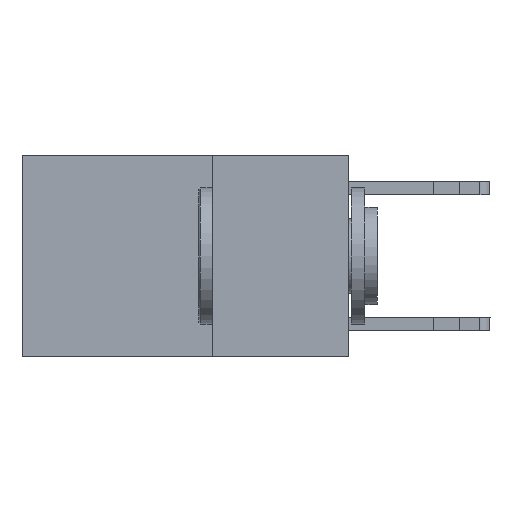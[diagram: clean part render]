
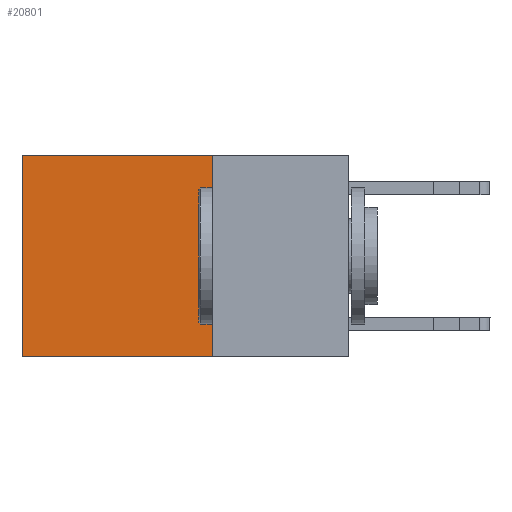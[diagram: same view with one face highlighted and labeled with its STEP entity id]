
A CAD part, left-side view. The second image highlights one B-rep face of the part: STEP entity #20801.
In plain terms, the highlighted planar face has unit normal (-1, 0, 0).
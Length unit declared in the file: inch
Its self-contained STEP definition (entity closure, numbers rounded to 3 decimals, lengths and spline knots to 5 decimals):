
#813 = ORIENTED_EDGE ( 'NONE', *, *, #5533, .F. ) ;
#1489 = VECTOR ( 'NONE', #18342, 39.37008 ) ;
#2137 = LINE ( 'NONE', #18968, #1489 ) ;
#3173 = VECTOR ( 'NONE', #22518, 39.37008 ) ;
#3373 = LINE ( 'NONE', #22597, #3173 ) ;
#4511 = CARTESIAN_POINT ( 'NONE',  ( 0.2625, 0.6, -0.37 ) ) ;
#5533 = EDGE_CURVE ( 'NONE', #21142, #20079, #14805, .T. ) ;
#5697 = CARTESIAN_POINT ( 'NONE',  ( 0.2625, 0.25, 0. ) ) ;
#5754 = DIRECTION ( 'NONE',  ( 0., 1., 0. ) ) ;
#5959 = EDGE_LOOP ( 'NONE', ( #14165, #813, #18058, #15944 ) ) ;
#6231 = CARTESIAN_POINT ( 'NONE',  ( 0.2625, 0.25, -0.37 ) ) ;
#6402 = FACE_OUTER_BOUND ( 'NONE', #5959, .T. ) ;
#8987 = CARTESIAN_POINT ( 'NONE',  ( 0.2625, 0.25, -0.37 ) ) ;
#12621 = VECTOR ( 'NONE', #21147, 39.37008 ) ;
#12795 = LINE ( 'NONE', #20859, #12621 ) ;
#14165 = ORIENTED_EDGE ( 'NONE', *, *, #17484, .T. ) ;
#14754 = VECTOR ( 'NONE', #5754, 39.37008 ) ;
#14805 = LINE ( 'NONE', #6231, #14754 ) ;
#15431 = EDGE_CURVE ( 'NONE', #21270, #23002, #3373, .T. ) ;
#15872 = CARTESIAN_POINT ( 'NONE',  ( 0.2625, 0.6, 0. ) ) ;
#15944 = ORIENTED_EDGE ( 'NONE', *, *, #15431, .T. ) ;
#16678 = EDGE_CURVE ( 'NONE', #21270, #21142, #12795, .T. ) ;
#17484 = EDGE_CURVE ( 'NONE', #23002, #20079, #2137, .T. ) ;
#17991 = DIRECTION ( 'NONE',  ( 0., 0., -1. ) ) ;
#18058 = ORIENTED_EDGE ( 'NONE', *, *, #16678, .F. ) ;
#18093 = DIRECTION ( 'NONE',  ( 1., 0., 0. ) ) ;
#18333 = PLANE ( 'NONE',  #19999 ) ;
#18342 = DIRECTION ( 'NONE',  ( 0., 0., -1. ) ) ;
#18540 = CARTESIAN_POINT ( 'NONE',  ( 0.2625, 0.25, 0. ) ) ;
#18968 = CARTESIAN_POINT ( 'NONE',  ( 0.2625, 0.6, 0. ) ) ;
#19999 = AXIS2_PLACEMENT_3D ( 'NONE', #18540, #18093, #17991 ) ;
#20079 = VERTEX_POINT ( 'NONE', #4511 ) ;
#20801 = ADVANCED_FACE ( 'NONE', ( #6402 ), #18333, .F. ) ;
#20859 = CARTESIAN_POINT ( 'NONE',  ( 0.2625, 0.25, 0. ) ) ;
#21142 = VERTEX_POINT ( 'NONE', #8987 ) ;
#21147 = DIRECTION ( 'NONE',  ( 0., 0., -1. ) ) ;
#21270 = VERTEX_POINT ( 'NONE', #5697 ) ;
#22518 = DIRECTION ( 'NONE',  ( 0., 1., 0. ) ) ;
#22597 = CARTESIAN_POINT ( 'NONE',  ( 0.2625, 0.25, 0. ) ) ;
#23002 = VERTEX_POINT ( 'NONE', #15872 ) ;
